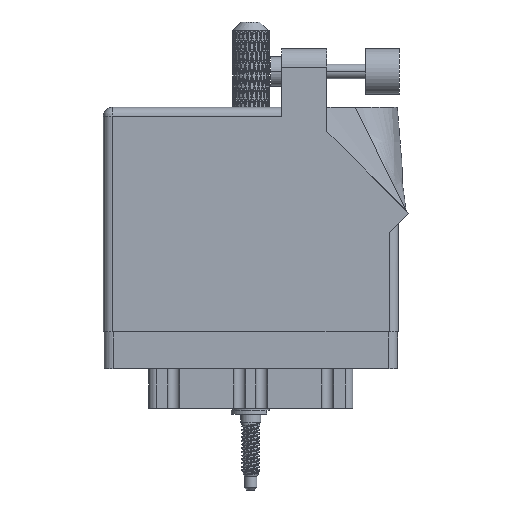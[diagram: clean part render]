
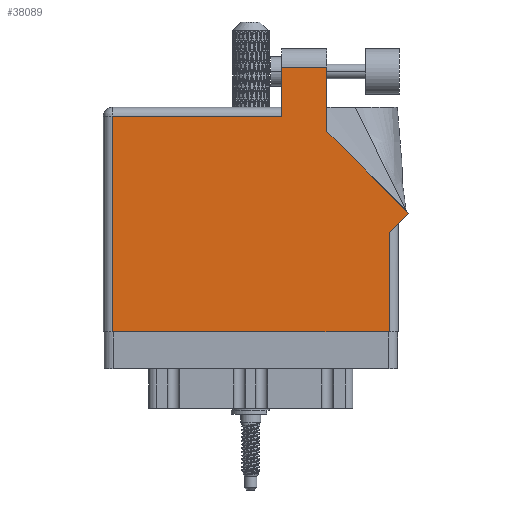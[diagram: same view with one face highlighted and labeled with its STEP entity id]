
A CAD part, front view. The second image highlights one B-rep face of the part: STEP entity #38089.
In plain terms, the highlighted face is planar.
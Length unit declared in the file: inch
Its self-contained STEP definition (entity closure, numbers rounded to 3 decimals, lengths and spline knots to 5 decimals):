
#293 = LINE ( 'NONE', #65817, #51425 ) ;
#439 = LINE ( 'NONE', #23681, #39394 ) ;
#675 = CARTESIAN_POINT ( 'NONE',  ( 0.062, 1.468, 0. ) ) ;
#1778 = ORIENTED_EDGE ( 'NONE', *, *, #90707, .T. ) ;
#7812 = LINE ( 'NONE', #40033, #13775 ) ;
#8015 = VERTEX_POINT ( 'NONE', #96778 ) ;
#9182 = ORIENTED_EDGE ( 'NONE', *, *, #9655, .T. ) ;
#9655 = EDGE_CURVE ( 'NONE', #96149, #90723, #7812, .T. ) ;
#11835 = EDGE_CURVE ( 'NONE', #89633, #96149, #53257, .T. ) ;
#12168 = ORIENTED_EDGE ( 'NONE', *, *, #102210, .T. ) ;
#13174 = CARTESIAN_POINT ( 'NONE',  ( 1.948, 0.675, 0. ) ) ;
#13775 = VECTOR ( 'NONE', #72301, 39.37008 ) ;
#15777 = VECTOR ( 'NONE', #49810, 39.37008 ) ;
#17050 = LINE ( 'NONE', #26019, #15777 ) ;
#17837 = EDGE_CURVE ( 'NONE', #90723, #75029, #293, .T. ) ;
#20343 = CARTESIAN_POINT ( 'NONE',  ( 1.217, 1.805, 0. ) ) ;
#21983 = CARTESIAN_POINT ( 'NONE',  ( 1.524, 1.36442, 0. ) ) ;
#22555 = DIRECTION ( 'NONE',  ( 0., 1., 0. ) ) ;
#23173 = DIRECTION ( 'NONE',  ( 0., -1., 0. ) ) ;
#23681 = CARTESIAN_POINT ( 'NONE',  ( 1.217, 1.53, 0. ) ) ;
#24066 = CARTESIAN_POINT ( 'NONE',  ( 0., 0., 0. ) ) ;
#24613 = CARTESIAN_POINT ( 'NONE',  ( 1.524, 1.805, 0. ) ) ;
#26019 = CARTESIAN_POINT ( 'NONE',  ( 0.062, 0., 0. ) ) ;
#31608 = EDGE_CURVE ( 'NONE', #70437, #53513, #84300, .T. ) ;
#32147 = CARTESIAN_POINT ( 'NONE',  ( 1.524, 1.36442, 0. ) ) ;
#32315 = VECTOR ( 'NONE', #44605, 39.37008 ) ;
#38089 = ADVANCED_FACE ( 'NONE', ( #104105 ), #39075, .F. ) ;
#39075 = PLANE ( 'NONE',  #78968 ) ;
#39394 = VECTOR ( 'NONE', #23173, 39.37008 ) ;
#40033 = CARTESIAN_POINT ( 'NONE',  ( 2.01, 0.737, 0. ) ) ;
#40975 = LINE ( 'NONE', #24066, #42837 ) ;
#42837 = VECTOR ( 'NONE', #81178, 39.37008 ) ;
#44126 = LINE ( 'NONE', #20343, #80246 ) ;
#44605 = DIRECTION ( 'NONE',  ( -1., 0., 0. ) ) ;
#44678 = ORIENTED_EDGE ( 'NONE', *, *, #17837, .T. ) ;
#46620 = VERTEX_POINT ( 'NONE', #71642 ) ;
#49810 = DIRECTION ( 'NONE',  ( 0., -1., 0. ) ) ;
#51425 = VECTOR ( 'NONE', #73217, 39.37008 ) ;
#52610 = DIRECTION ( 'NONE',  ( -1., 0., 0. ) ) ;
#53189 = EDGE_CURVE ( 'NONE', #75029, #101991, #94418, .T. ) ;
#53257 = LINE ( 'NONE', #87584, #103432 ) ;
#53513 = VERTEX_POINT ( 'NONE', #675 ) ;
#53928 = EDGE_LOOP ( 'NONE', ( #82846, #12168, #1778, #55338, #91188, #62731, #66221, #9182, #44678 ) ) ;
#54244 = DIRECTION ( 'NONE',  ( 0., 1., 0. ) ) ;
#55338 = ORIENTED_EDGE ( 'NONE', *, *, #31608, .T. ) ;
#58933 = CARTESIAN_POINT ( 'NONE',  ( 0., 1.468, 0. ) ) ;
#59691 = CARTESIAN_POINT ( 'NONE',  ( 1.948, 0., 0. ) ) ;
#62731 = ORIENTED_EDGE ( 'NONE', *, *, #65768, .T. ) ;
#63940 = DIRECTION ( 'NONE',  ( -1., 0., 0. ) ) ;
#64943 = EDGE_CURVE ( 'NONE', #53513, #8015, #17050, .T. ) ;
#65768 = EDGE_CURVE ( 'NONE', #8015, #89633, #40975, .T. ) ;
#65817 = CARTESIAN_POINT ( 'NONE',  ( 2.08071, 0.80771, 0. ) ) ;
#66221 = ORIENTED_EDGE ( 'NONE', *, *, #11835, .T. ) ;
#70437 = VERTEX_POINT ( 'NONE', #96366 ) ;
#71347 = DIRECTION ( 'NONE',  ( 0., 0., -1. ) ) ;
#71642 = CARTESIAN_POINT ( 'NONE',  ( 1.217, 1.805, 0. ) ) ;
#72301 = DIRECTION ( 'NONE',  ( 0.707, 0.707, 0. ) ) ;
#73217 = DIRECTION ( 'NONE',  ( -0.707, 0.707, 0. ) ) ;
#75029 = VERTEX_POINT ( 'NONE', #32147 ) ;
#78968 = AXIS2_PLACEMENT_3D ( 'NONE', #95664, #71347, #63940 ) ;
#80246 = VECTOR ( 'NONE', #52610, 39.37008 ) ;
#81178 = DIRECTION ( 'NONE',  ( 1., 0., 0. ) ) ;
#82846 = ORIENTED_EDGE ( 'NONE', *, *, #53189, .T. ) ;
#84300 = LINE ( 'NONE', #58933, #32315 ) ;
#87584 = CARTESIAN_POINT ( 'NONE',  ( 1.948, 0.737, 0. ) ) ;
#89633 = VERTEX_POINT ( 'NONE', #59691 ) ;
#90707 = EDGE_CURVE ( 'NONE', #46620, #70437, #439, .T. ) ;
#90723 = VERTEX_POINT ( 'NONE', #98185 ) ;
#91188 = ORIENTED_EDGE ( 'NONE', *, *, #64943, .T. ) ;
#94418 = LINE ( 'NONE', #21983, #94478 ) ;
#94478 = VECTOR ( 'NONE', #54244, 39.37008 ) ;
#95664 = CARTESIAN_POINT ( 'NONE',  ( 0., 1.53, 0. ) ) ;
#96149 = VERTEX_POINT ( 'NONE', #13174 ) ;
#96366 = CARTESIAN_POINT ( 'NONE',  ( 1.217, 1.468, 0. ) ) ;
#96778 = CARTESIAN_POINT ( 'NONE',  ( 0.062, 0., 0. ) ) ;
#98185 = CARTESIAN_POINT ( 'NONE',  ( 2.08071, 0.80771, 0. ) ) ;
#101991 = VERTEX_POINT ( 'NONE', #24613 ) ;
#102210 = EDGE_CURVE ( 'NONE', #101991, #46620, #44126, .T. ) ;
#103432 = VECTOR ( 'NONE', #22555, 39.37008 ) ;
#104105 = FACE_OUTER_BOUND ( 'NONE', #53928, .T. ) ;
